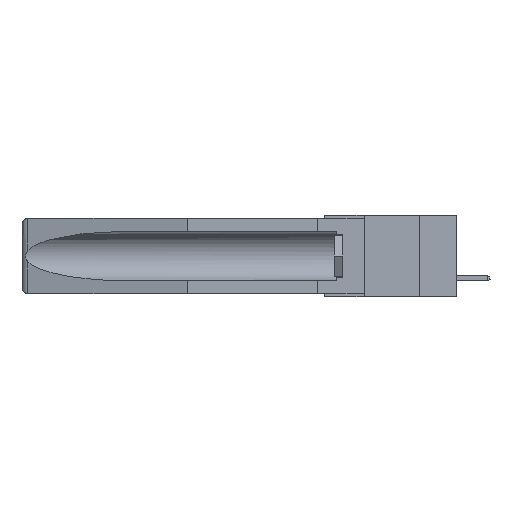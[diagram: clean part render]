
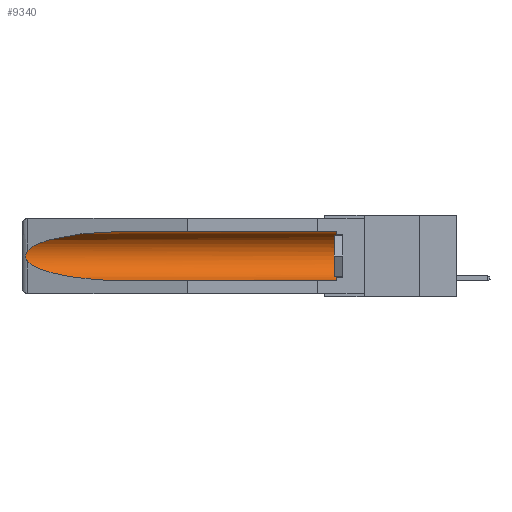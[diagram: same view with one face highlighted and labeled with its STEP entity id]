
A CAD part, left-side view. The second image highlights one B-rep face of the part: STEP entity #9340.
In plain terms, the highlighted cylindrical face has radius 2.857 mm (diameter 5.715 mm), a partial arc.
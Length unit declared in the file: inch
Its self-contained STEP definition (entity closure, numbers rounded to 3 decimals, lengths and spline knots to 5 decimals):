
#596 = EDGE_CURVE ( 'NONE', #16697, #10708, #3782, .T. ) ;
#763 = DIRECTION ( 'NONE',  ( 0., 0., 1. ) ) ;
#1658 = CARTESIAN_POINT ( 'NONE',  ( 0.155, -0.30754, -0.284 ) ) ;
#1848 = CARTESIAN_POINT ( 'NONE',  ( 0.2675, 1.53308, -0.16763 ) ) ;
#1865 = VERTEX_POINT ( 'NONE', #12332 ) ;
#2914 = VERTEX_POINT ( 'NONE', #28239 ) ;
#3248 =( BOUNDED_CURVE ( )  B_SPLINE_CURVE ( 3, ( #20289, #20595, #18135, #7294 ),
 .UNSPECIFIED., .F., .T. ) 
 B_SPLINE_CURVE_WITH_KNOTS ( ( 4, 4 ),
 ( 0.1948, 1.5708 ),
 .UNSPECIFIED. ) 
 CURVE ( )  GEOMETRIC_REPRESENTATION_ITEM ( )  RATIONAL_B_SPLINE_CURVE ( ( 1., 0.848, 0.848, 1. ) ) 
 REPRESENTATION_ITEM ( '' )  );
#3782 = CIRCLE ( 'NONE', #24249, 0.1125 ) ;
#3893 = LINE ( 'NONE', #5566, #9086 ) ;
#4029 = CARTESIAN_POINT ( 'NONE',  ( 0.26655, 1.53094, -0.18657 ) ) ;
#4128 = CARTESIAN_POINT ( 'NONE',  ( 0.155, 1.07973, -0.059 ) ) ;
#5566 = CARTESIAN_POINT ( 'NONE',  ( 0.155, -0.30754, -0.059 ) ) ;
#6099 = CARTESIAN_POINT ( 'NONE',  ( 0.2673, 1.5327, -0.16383 ) ) ;
#6346 = EDGE_LOOP ( 'NONE', ( #26861, #13122, #28060, #15090, #8028, #22988 ) ) ;
#7294 = CARTESIAN_POINT ( 'NONE',  ( 0.155, 1.07973, -0.284 ) ) ;
#7643 = CARTESIAN_POINT ( 'NONE',  ( 0.155, 0.126, -0.1715 ) ) ;
#8028 = ORIENTED_EDGE ( 'NONE', *, *, #596, .T. ) ;
#8102 = CARTESIAN_POINT ( 'NONE',  ( 0.2675, 1.53308, -0.17534 ) ) ;
#8312 = CARTESIAN_POINT ( 'NONE',  ( 0.26537, 1.52718, -0.14972 ) ) ;
#9086 = VECTOR ( 'NONE', #25795, 39.37008 ) ;
#9340 = ADVANCED_FACE ( 'NONE', ( #23742 ), #24098, .F. ) ;
#10158 = EDGE_CURVE ( 'NONE', #1865, #24785, #3248, .T. ) ;
#10708 = VERTEX_POINT ( 'NONE', #13635 ) ;
#12011 = DIRECTION ( 'NONE',  ( 0., -1., 0. ) ) ;
#12246 = AXIS2_PLACEMENT_3D ( 'NONE', #27385, #27675, #763 ) ;
#12314 =( BOUNDED_CURVE ( )  B_SPLINE_CURVE ( 3, ( #4128, #21931, #14790, #8312 ),
 .UNSPECIFIED., .F., .F. ) 
 B_SPLINE_CURVE_WITH_KNOTS ( ( 4, 4 ),
 ( 4.71239, 6.08839 ),
 .UNSPECIFIED. ) 
 CURVE ( )  GEOMETRIC_REPRESENTATION_ITEM ( )  RATIONAL_B_SPLINE_CURVE ( ( 1., 0.848, 0.848, 1. ) ) 
 REPRESENTATION_ITEM ( '' )  );
#12332 = CARTESIAN_POINT ( 'NONE',  ( 0.26537, 1.52718, -0.19328 ) ) ;
#12752 = CARTESIAN_POINT ( 'NONE',  ( 0.2673, 1.53269, -0.17917 ) ) ;
#13122 = ORIENTED_EDGE ( 'NONE', *, *, #17208, .T. ) ;
#13635 = CARTESIAN_POINT ( 'NONE',  ( 0.155, 0.126, -0.059 ) ) ;
#13653 = EDGE_CURVE ( 'NONE', #2914, #19891, #12314, .T. ) ;
#14433 = B_SPLINE_CURVE_WITH_KNOTS ( 'NONE', 3,
 ( #26339, #21433, #26137, #6099, #1848, #8102, #12752, #4029, #23680, #19250 ),
 .UNSPECIFIED., .F., .F.,
 ( 4, 2, 2, 2, 4 ),
 ( 0., 0.00029, 0.00058, 0.00087, 0.00117 ),
 .UNSPECIFIED. ) ;
#14790 = CARTESIAN_POINT ( 'NONE',  ( 0.25451, 1.48313, -0.09465 ) ) ;
#15090 = ORIENTED_EDGE ( 'NONE', *, *, #17271, .F. ) ;
#16460 = EDGE_CURVE ( 'NONE', #10708, #2914, #3893, .T. ) ;
#16697 = VERTEX_POINT ( 'NONE', #17425 ) ;
#17208 = EDGE_CURVE ( 'NONE', #19891, #1865, #14433, .T. ) ;
#17271 = EDGE_CURVE ( 'NONE', #16697, #24785, #22279, .T. ) ;
#17303 = DIRECTION ( 'NONE',  ( 0., 1., 0. ) ) ;
#17425 = CARTESIAN_POINT ( 'NONE',  ( 0.155, 0.126, -0.284 ) ) ;
#18135 = CARTESIAN_POINT ( 'NONE',  ( 0.21114, 1.30732, -0.284 ) ) ;
#18868 = DIRECTION ( 'NONE',  ( 0., 0., 1. ) ) ;
#19250 = CARTESIAN_POINT ( 'NONE',  ( 0.26537, 1.52718, -0.19328 ) ) ;
#19891 = VERTEX_POINT ( 'NONE', #23179 ) ;
#20289 = CARTESIAN_POINT ( 'NONE',  ( 0.26537, 1.52718, -0.19328 ) ) ;
#20595 = CARTESIAN_POINT ( 'NONE',  ( 0.25451, 1.48313, -0.24835 ) ) ;
#21433 = CARTESIAN_POINT ( 'NONE',  ( 0.26597, 1.52961, -0.15275 ) ) ;
#21931 = CARTESIAN_POINT ( 'NONE',  ( 0.21114, 1.30732, -0.059 ) ) ;
#22279 = LINE ( 'NONE', #1658, #24022 ) ;
#22988 = ORIENTED_EDGE ( 'NONE', *, *, #16460, .T. ) ;
#23179 = CARTESIAN_POINT ( 'NONE',  ( 0.26537, 1.52718, -0.14972 ) ) ;
#23680 = CARTESIAN_POINT ( 'NONE',  ( 0.26597, 1.5296, -0.19026 ) ) ;
#23742 = FACE_OUTER_BOUND ( 'NONE', #6346, .T. ) ;
#24022 = VECTOR ( 'NONE', #17303, 39.37008 ) ;
#24098 = CYLINDRICAL_SURFACE ( 'NONE', #12246, 0.1125 ) ;
#24249 = AXIS2_PLACEMENT_3D ( 'NONE', #7643, #12011, #18868 ) ;
#24785 = VERTEX_POINT ( 'NONE', #24863 ) ;
#24863 = CARTESIAN_POINT ( 'NONE',  ( 0.155, 1.07973, -0.284 ) ) ;
#25795 = DIRECTION ( 'NONE',  ( 0., 1., 0. ) ) ;
#26137 = CARTESIAN_POINT ( 'NONE',  ( 0.26654, 1.53092, -0.15636 ) ) ;
#26339 = CARTESIAN_POINT ( 'NONE',  ( 0.26537, 1.52718, -0.14972 ) ) ;
#26861 = ORIENTED_EDGE ( 'NONE', *, *, #13653, .T. ) ;
#27385 = CARTESIAN_POINT ( 'NONE',  ( 0.155, -0.30754, -0.1715 ) ) ;
#27675 = DIRECTION ( 'NONE',  ( 0., 1., 0. ) ) ;
#28060 = ORIENTED_EDGE ( 'NONE', *, *, #10158, .T. ) ;
#28239 = CARTESIAN_POINT ( 'NONE',  ( 0.155, 1.07973, -0.059 ) ) ;
